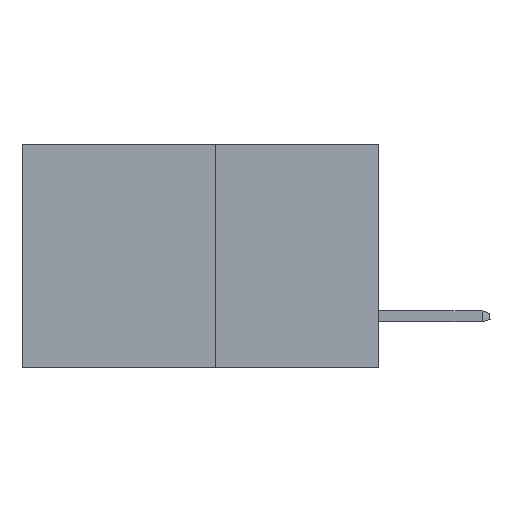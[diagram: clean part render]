
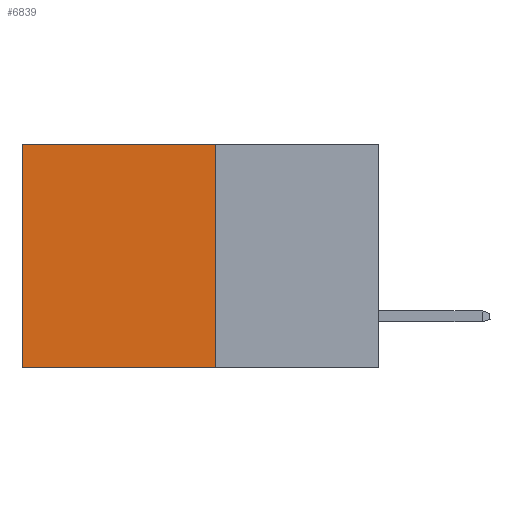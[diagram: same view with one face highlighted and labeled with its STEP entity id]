
A CAD part, left-side view. The second image highlights one B-rep face of the part: STEP entity #6839.
In plain terms, the highlighted planar face has unit normal (-1, 0, 0).
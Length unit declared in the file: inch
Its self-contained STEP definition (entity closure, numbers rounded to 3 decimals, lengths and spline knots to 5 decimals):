
#39 = VERTEX_POINT ( 'NONE', #246 ) ;
#246 = CARTESIAN_POINT ( 'NONE',  ( 0.277, 0.27, 0. ) ) ;
#503 = PLANE ( 'NONE',  #11731 ) ;
#1597 = CARTESIAN_POINT ( 'NONE',  ( 0.277, 0.59, -0.37 ) ) ;
#1895 = LINE ( 'NONE', #10472, #15881 ) ;
#1987 = DIRECTION ( 'NONE',  ( 0., 0., -1. ) ) ;
#1994 = DIRECTION ( 'NONE',  ( 0., 1., 0. ) ) ;
#2176 = CARTESIAN_POINT ( 'NONE',  ( 0.277, 0.59, 0. ) ) ;
#2275 = EDGE_CURVE ( 'NONE', #4927, #12987, #2946, .T. ) ;
#2281 = EDGE_LOOP ( 'NONE', ( #10990, #10368, #12383, #4539 ) ) ;
#2946 = LINE ( 'NONE', #15947, #9601 ) ;
#3509 = LINE ( 'NONE', #16459, #14271 ) ;
#4539 = ORIENTED_EDGE ( 'NONE', *, *, #14350, .T. ) ;
#4927 = VERTEX_POINT ( 'NONE', #7669 ) ;
#6787 = DIRECTION ( 'NONE',  ( 0., 0., -1. ) ) ;
#6839 = ADVANCED_FACE ( 'NONE', ( #12292 ), #503, .F. ) ;
#7669 = CARTESIAN_POINT ( 'NONE',  ( 0.277, 0.27, -0.37 ) ) ;
#8649 = LINE ( 'NONE', #17815, #12376 ) ;
#8833 = EDGE_CURVE ( 'NONE', #39, #4927, #3509, .T. ) ;
#9601 = VECTOR ( 'NONE', #16860, 39.37008 ) ;
#10368 = ORIENTED_EDGE ( 'NONE', *, *, #2275, .F. ) ;
#10461 = DIRECTION ( 'NONE',  ( 1., 0., 0. ) ) ;
#10472 = CARTESIAN_POINT ( 'NONE',  ( 0.277, 0.27, 0. ) ) ;
#10990 = ORIENTED_EDGE ( 'NONE', *, *, #12290, .T. ) ;
#11731 = AXIS2_PLACEMENT_3D ( 'NONE', #17300, #10461, #1987 ) ;
#12147 = VERTEX_POINT ( 'NONE', #2176 ) ;
#12290 = EDGE_CURVE ( 'NONE', #12147, #12987, #8649, .T. ) ;
#12292 = FACE_OUTER_BOUND ( 'NONE', #2281, .T. ) ;
#12371 = DIRECTION ( 'NONE',  ( 0., 0., -1. ) ) ;
#12376 = VECTOR ( 'NONE', #6787, 39.37008 ) ;
#12383 = ORIENTED_EDGE ( 'NONE', *, *, #8833, .F. ) ;
#12987 = VERTEX_POINT ( 'NONE', #1597 ) ;
#14271 = VECTOR ( 'NONE', #12371, 39.37008 ) ;
#14350 = EDGE_CURVE ( 'NONE', #39, #12147, #1895, .T. ) ;
#15881 = VECTOR ( 'NONE', #1994, 39.37008 ) ;
#15947 = CARTESIAN_POINT ( 'NONE',  ( 0.277, 0.27, -0.37 ) ) ;
#16459 = CARTESIAN_POINT ( 'NONE',  ( 0.277, 0.27, -0.37 ) ) ;
#16860 = DIRECTION ( 'NONE',  ( 0., 1., 0. ) ) ;
#17300 = CARTESIAN_POINT ( 'NONE',  ( 0.277, 0.27, -0.37 ) ) ;
#17815 = CARTESIAN_POINT ( 'NONE',  ( 0.277, 0.59, -0.37 ) ) ;
